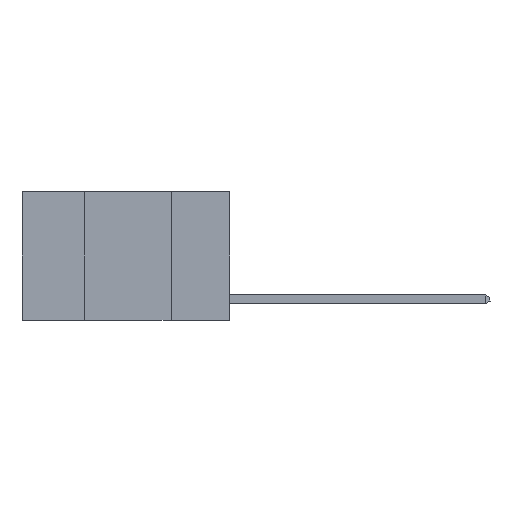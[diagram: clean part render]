
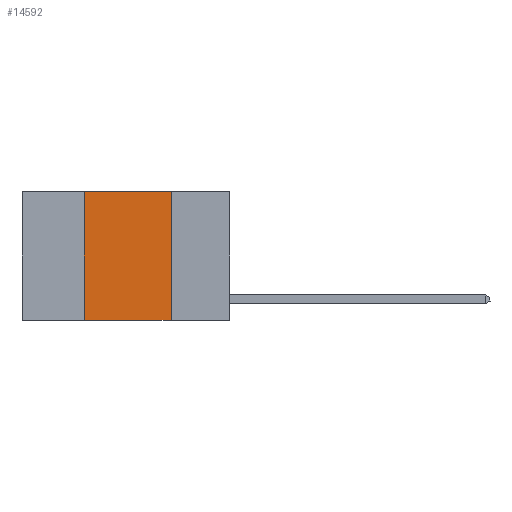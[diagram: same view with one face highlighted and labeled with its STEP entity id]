
A CAD part, left-side view. The second image highlights one B-rep face of the part: STEP entity #14592.
In plain terms, the highlighted planar face has unit normal (-1, 0, 0).
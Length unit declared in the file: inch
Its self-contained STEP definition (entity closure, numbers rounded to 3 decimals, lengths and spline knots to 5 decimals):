
#140 = DIRECTION ( 'NONE',  ( 0., 0., 1. ) ) ;
#245 = DIRECTION ( 'NONE',  ( 1., 0., 0. ) ) ;
#1805 = EDGE_CURVE ( 'NONE', #19567, #6926, #13973, .T. ) ;
#2283 = AXIS2_PLACEMENT_3D ( 'NONE', #6741, #245, #2518 ) ;
#2518 = DIRECTION ( 'NONE',  ( 0., 0., -1. ) ) ;
#2991 = CARTESIAN_POINT ( 'NONE',  ( 0., 0.17, 0. ) ) ;
#3549 = VERTEX_POINT ( 'NONE', #20357 ) ;
#3948 = VECTOR ( 'NONE', #19195, 39.37008 ) ;
#5789 = ORIENTED_EDGE ( 'NONE', *, *, #26941, .F. ) ;
#5920 = ORIENTED_EDGE ( 'NONE', *, *, #15676, .F. ) ;
#5989 = VECTOR ( 'NONE', #140, 39.37008 ) ;
#6173 = DIRECTION ( 'NONE',  ( 0., 0., -1. ) ) ;
#6412 = VERTEX_POINT ( 'NONE', #2991 ) ;
#6741 = CARTESIAN_POINT ( 'NONE',  ( 0., 0.6, 0. ) ) ;
#6926 = VERTEX_POINT ( 'NONE', #17077 ) ;
#7042 = PLANE ( 'NONE',  #2283 ) ;
#9252 = CARTESIAN_POINT ( 'NONE',  ( 0., 0.42, 0. ) ) ;
#10375 = CARTESIAN_POINT ( 'NONE',  ( 0., 0.6, -0.37 ) ) ;
#11545 = EDGE_CURVE ( 'NONE', #3549, #6412, #21176, .T. ) ;
#12017 = LINE ( 'NONE', #9252, #5989 ) ;
#12033 = CARTESIAN_POINT ( 'NONE',  ( 0., 0.42, -0.37 ) ) ;
#12544 = EDGE_LOOP ( 'NONE', ( #5920, #23828, #5789, #14488 ) ) ;
#13973 = LINE ( 'NONE', #10375, #15392 ) ;
#14488 = ORIENTED_EDGE ( 'NONE', *, *, #1805, .T. ) ;
#14592 = ADVANCED_FACE ( 'NONE', ( #28492 ), #7042, .F. ) ;
#14611 = CARTESIAN_POINT ( 'NONE',  ( 0., 0.6, 0. ) ) ;
#15208 = LINE ( 'NONE', #17320, #15543 ) ;
#15392 = VECTOR ( 'NONE', #21670, 39.37008 ) ;
#15543 = VECTOR ( 'NONE', #6173, 39.37008 ) ;
#15676 = EDGE_CURVE ( 'NONE', #6412, #6926, #15208, .T. ) ;
#17077 = CARTESIAN_POINT ( 'NONE',  ( 0., 0.17, -0.37 ) ) ;
#17320 = CARTESIAN_POINT ( 'NONE',  ( 0., 0.17, 0. ) ) ;
#19195 = DIRECTION ( 'NONE',  ( 0., -1., 0. ) ) ;
#19567 = VERTEX_POINT ( 'NONE', #12033 ) ;
#20357 = CARTESIAN_POINT ( 'NONE',  ( 0., 0.42, 0. ) ) ;
#21176 = LINE ( 'NONE', #14611, #3948 ) ;
#21670 = DIRECTION ( 'NONE',  ( 0., -1., 0. ) ) ;
#23828 = ORIENTED_EDGE ( 'NONE', *, *, #11545, .F. ) ;
#26941 = EDGE_CURVE ( 'NONE', #19567, #3549, #12017, .T. ) ;
#28492 = FACE_OUTER_BOUND ( 'NONE', #12544, .T. ) ;
